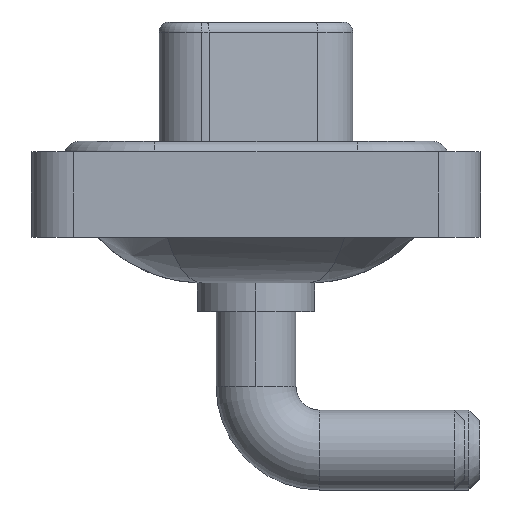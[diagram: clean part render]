
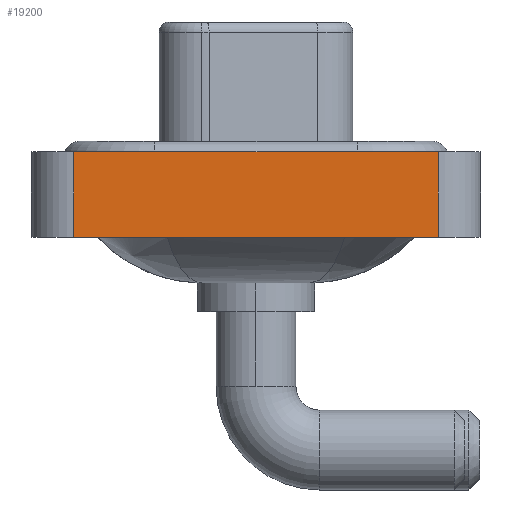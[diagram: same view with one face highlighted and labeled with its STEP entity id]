
A CAD part, left-side view. The second image highlights one B-rep face of the part: STEP entity #19200.
In plain terms, the highlighted planar face has unit normal (-1, 0, 0).
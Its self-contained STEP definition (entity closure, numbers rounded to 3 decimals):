
#426 = EDGE_CURVE ( 'NONE', #15513, #12842, #14172, .T. ) ;
#482 = ORIENTED_EDGE ( 'NONE', *, *, #11404, .F. ) ;
#1120 = DIRECTION ( 'NONE',  ( 0., -1., 0. ) ) ;
#1837 = ORIENTED_EDGE ( 'NONE', *, *, #2461, .T. ) ;
#2461 = EDGE_CURVE ( 'NONE', #11225, #15513, #5272, .T. ) ;
#2812 = DIRECTION ( 'NONE',  ( 0., 0., 1. ) ) ;
#3236 = VECTOR ( 'NONE', #12251, 1000. ) ;
#4012 = CARTESIAN_POINT ( 'NONE',  ( -7.3, -8.55, 0.4 ) ) ;
#4276 = EDGE_CURVE ( 'NONE', #6382, #12842, #13934, .T. ) ;
#5272 = LINE ( 'NONE', #5565, #8993 ) ;
#5369 = ORIENTED_EDGE ( 'NONE', *, *, #426, .T. ) ;
#5565 = CARTESIAN_POINT ( 'NONE',  ( -7.3, -8.55, -3.6 ) ) ;
#5889 = PLANE ( 'NONE',  #19249 ) ;
#6382 = VERTEX_POINT ( 'NONE', #18120 ) ;
#7158 = FACE_OUTER_BOUND ( 'NONE', #8205, .T. ) ;
#7771 = CARTESIAN_POINT ( 'NONE',  ( -7.3, 8.55, -3.6 ) ) ;
#8205 = EDGE_LOOP ( 'NONE', ( #5369, #15615, #482, #1837 ) ) ;
#8332 = CARTESIAN_POINT ( 'NONE',  ( -7.3, 8.55, -3.6 ) ) ;
#8993 = VECTOR ( 'NONE', #1120, 1000. ) ;
#11225 = VERTEX_POINT ( 'NONE', #7771 ) ;
#11283 = LINE ( 'NONE', #8332, #14213 ) ;
#11404 = EDGE_CURVE ( 'NONE', #11225, #6382, #11283, .T. ) ;
#11608 = DIRECTION ( 'NONE',  ( 0., -1., 0. ) ) ;
#12251 = DIRECTION ( 'NONE',  ( 0., 0., 1. ) ) ;
#12347 = CARTESIAN_POINT ( 'NONE',  ( -7.3, -8.55, -3.6 ) ) ;
#12836 = DIRECTION ( 'NONE',  ( 0., 0., 1. ) ) ;
#12842 = VERTEX_POINT ( 'NONE', #16093 ) ;
#13303 = DIRECTION ( 'NONE',  ( -1., 0., 0. ) ) ;
#13934 = LINE ( 'NONE', #4012, #15025 ) ;
#14172 = LINE ( 'NONE', #12347, #3236 ) ;
#14213 = VECTOR ( 'NONE', #12836, 1000. ) ;
#14780 = CARTESIAN_POINT ( 'NONE',  ( -7.3, -8.55, -3.6 ) ) ;
#15025 = VECTOR ( 'NONE', #11608, 1000. ) ;
#15513 = VERTEX_POINT ( 'NONE', #19020 ) ;
#15615 = ORIENTED_EDGE ( 'NONE', *, *, #4276, .F. ) ;
#16093 = CARTESIAN_POINT ( 'NONE',  ( -7.3, -8.55, 0.4 ) ) ;
#18120 = CARTESIAN_POINT ( 'NONE',  ( -7.3, 8.55, 0.4 ) ) ;
#19020 = CARTESIAN_POINT ( 'NONE',  ( -7.3, -8.55, -3.6 ) ) ;
#19200 = ADVANCED_FACE ( 'NONE', ( #7158 ), #5889, .T. ) ;
#19249 = AXIS2_PLACEMENT_3D ( 'NONE', #14780, #13303, #2812 ) ;
